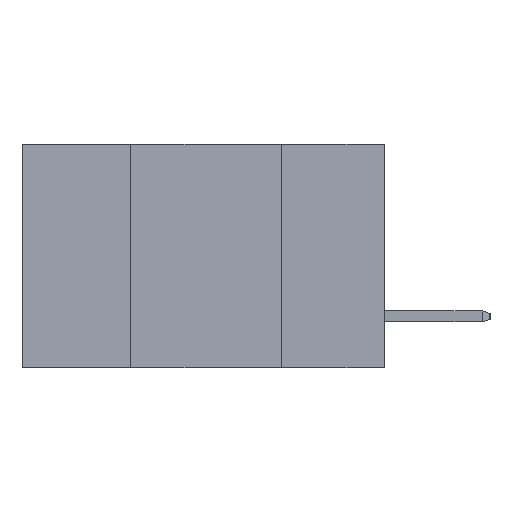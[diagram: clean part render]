
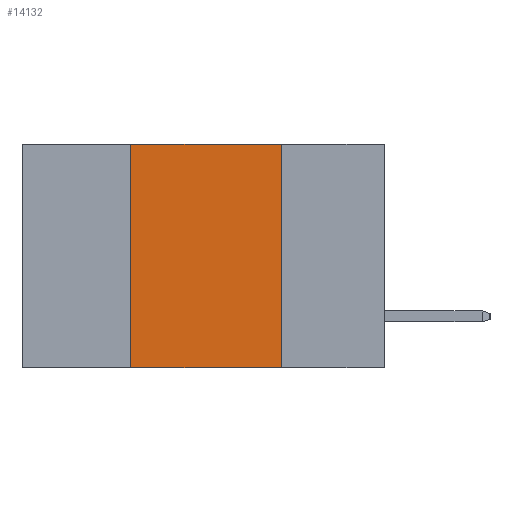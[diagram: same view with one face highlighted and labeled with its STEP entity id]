
A CAD part, left-side view. The second image highlights one B-rep face of the part: STEP entity #14132.
In plain terms, the highlighted planar face has unit normal (-1, 0, 0).
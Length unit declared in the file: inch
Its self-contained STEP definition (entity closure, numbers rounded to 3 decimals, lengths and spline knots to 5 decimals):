
#284 = ORIENTED_EDGE ( 'NONE', *, *, #6050, .F. ) ;
#435 = VECTOR ( 'NONE', #701, 39.37008 ) ;
#540 = CARTESIAN_POINT ( 'NONE',  ( 0., 0.42, 0. ) ) ;
#701 = DIRECTION ( 'NONE',  ( 0., 0., 1. ) ) ;
#984 = FACE_OUTER_BOUND ( 'NONE', #3699, .T. ) ;
#1045 = CARTESIAN_POINT ( 'NONE',  ( 0., 0.17, 0. ) ) ;
#1564 = PLANE ( 'NONE',  #9134 ) ;
#1781 = EDGE_CURVE ( 'NONE', #14533, #3853, #14024, .T. ) ;
#2048 = ORIENTED_EDGE ( 'NONE', *, *, #14248, .F. ) ;
#2312 = VECTOR ( 'NONE', #6359, 39.37008 ) ;
#2753 = DIRECTION ( 'NONE',  ( 1., 0., 0. ) ) ;
#2811 = VECTOR ( 'NONE', #11120, 39.37008 ) ;
#3093 = VERTEX_POINT ( 'NONE', #11006 ) ;
#3258 = EDGE_CURVE ( 'NONE', #3093, #8685, #14816, .T. ) ;
#3323 = CARTESIAN_POINT ( 'NONE',  ( 0., 0.17, -0.37 ) ) ;
#3699 = EDGE_LOOP ( 'NONE', ( #2048, #14465, #284, #9738 ) ) ;
#3853 = VERTEX_POINT ( 'NONE', #3323 ) ;
#5970 = CARTESIAN_POINT ( 'NONE',  ( 0., 0.6, -0.37 ) ) ;
#6050 = EDGE_CURVE ( 'NONE', #14533, #3093, #6691, .T. ) ;
#6359 = DIRECTION ( 'NONE',  ( 0., 0., -1. ) ) ;
#6691 = LINE ( 'NONE', #540, #435 ) ;
#7517 = CARTESIAN_POINT ( 'NONE',  ( 0., 0.17, 0. ) ) ;
#8420 = LINE ( 'NONE', #7517, #2312 ) ;
#8685 = VERTEX_POINT ( 'NONE', #1045 ) ;
#9134 = AXIS2_PLACEMENT_3D ( 'NONE', #12962, #2753, #10752 ) ;
#9738 = ORIENTED_EDGE ( 'NONE', *, *, #1781, .T. ) ;
#9945 = CARTESIAN_POINT ( 'NONE',  ( 0., 0.6, 0. ) ) ;
#10752 = DIRECTION ( 'NONE',  ( 0., 0., -1. ) ) ;
#11006 = CARTESIAN_POINT ( 'NONE',  ( 0., 0.42, 0. ) ) ;
#11070 = VECTOR ( 'NONE', #11929, 39.37008 ) ;
#11120 = DIRECTION ( 'NONE',  ( 0., -1., 0. ) ) ;
#11429 = CARTESIAN_POINT ( 'NONE',  ( 0., 0.42, -0.37 ) ) ;
#11929 = DIRECTION ( 'NONE',  ( 0., -1., 0. ) ) ;
#12962 = CARTESIAN_POINT ( 'NONE',  ( 0., 0.6, 0. ) ) ;
#14024 = LINE ( 'NONE', #5970, #11070 ) ;
#14132 = ADVANCED_FACE ( 'NONE', ( #984 ), #1564, .F. ) ;
#14248 = EDGE_CURVE ( 'NONE', #8685, #3853, #8420, .T. ) ;
#14465 = ORIENTED_EDGE ( 'NONE', *, *, #3258, .F. ) ;
#14533 = VERTEX_POINT ( 'NONE', #11429 ) ;
#14816 = LINE ( 'NONE', #9945, #2811 ) ;
